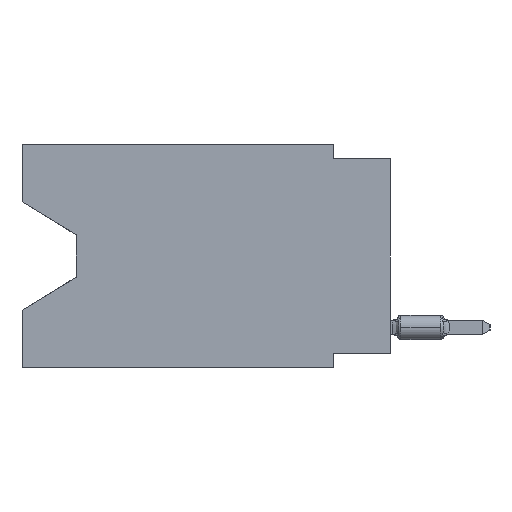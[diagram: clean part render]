
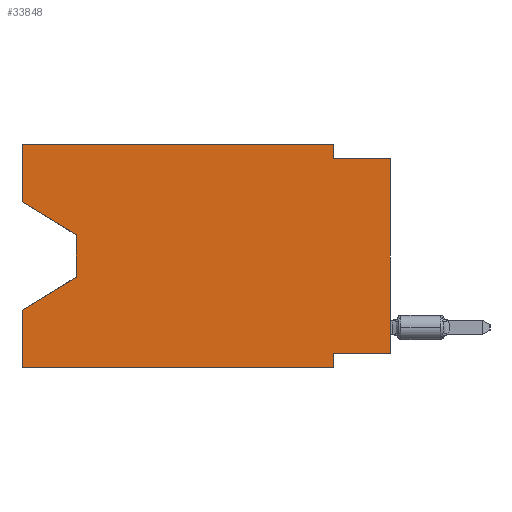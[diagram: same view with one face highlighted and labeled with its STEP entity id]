
A CAD part, left-side view. The second image highlights one B-rep face of the part: STEP entity #33848.
In plain terms, the highlighted planar face has unit normal (-1, 0, 0).
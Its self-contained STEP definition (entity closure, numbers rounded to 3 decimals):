
#257 = CARTESIAN_POINT ( 'NONE',  ( 0., 13.97, -5.893 ) ) ;
#1339 = VERTEX_POINT ( 'NONE', #38649 ) ;
#1725 = DIRECTION ( 'NONE',  ( 0., 0., -1. ) ) ;
#2882 = ORIENTED_EDGE ( 'NONE', *, *, #54597, .F. ) ;
#3100 = CARTESIAN_POINT ( 'NONE',  ( 0., 16.383, 0. ) ) ;
#3174 = VERTEX_POINT ( 'NONE', #54412 ) ;
#3651 = LINE ( 'NONE', #21540, #55730 ) ;
#3678 = DIRECTION ( 'NONE',  ( 0., 0., -1. ) ) ;
#3835 = CARTESIAN_POINT ( 'NONE',  ( 0., 0., -9.271 ) ) ;
#3837 = CARTESIAN_POINT ( 'NONE',  ( 0., 16.383, -2.546 ) ) ;
#4799 = VECTOR ( 'NONE', #37117, 1000. ) ;
#4942 = DIRECTION ( 'NONE',  ( 0., 0., -1. ) ) ;
#4967 = PLANE ( 'NONE',  #34024 ) ;
#5284 = CARTESIAN_POINT ( 'NONE',  ( 0., 16.383, 0. ) ) ;
#5517 = DIRECTION ( 'NONE',  ( 0., 0., -1. ) ) ;
#5522 = LINE ( 'NONE', #55066, #19893 ) ;
#5635 = ORIENTED_EDGE ( 'NONE', *, *, #6191, .T. ) ;
#6114 = DIRECTION ( 'NONE',  ( 1., 0., 0. ) ) ;
#6191 = EDGE_CURVE ( 'NONE', #15219, #54762, #33074, .T. ) ;
#6906 = VERTEX_POINT ( 'NONE', #33148 ) ;
#7361 = VECTOR ( 'NONE', #35498, 1000. ) ;
#8407 = LINE ( 'NONE', #13115, #34169 ) ;
#9062 = LINE ( 'NONE', #257, #13951 ) ;
#9277 = DIRECTION ( 'NONE',  ( 0., -1., 0. ) ) ;
#9693 = VECTOR ( 'NONE', #36617, 1000. ) ;
#9727 = EDGE_CURVE ( 'NONE', #12038, #9854, #42614, .T. ) ;
#9854 = VERTEX_POINT ( 'NONE', #57564 ) ;
#11542 = DIRECTION ( 'NONE',  ( 0., 0., 1. ) ) ;
#11933 = ORIENTED_EDGE ( 'NONE', *, *, #32653, .F. ) ;
#12038 = VERTEX_POINT ( 'NONE', #34923 ) ;
#12649 = LINE ( 'NONE', #3837, #7361 ) ;
#13115 = CARTESIAN_POINT ( 'NONE',  ( 0., 16.383, -9.906 ) ) ;
#13951 = VECTOR ( 'NONE', #54199, 1000. ) ;
#14295 = EDGE_CURVE ( 'NONE', #41225, #6906, #5522, .T. ) ;
#14967 = ORIENTED_EDGE ( 'NONE', *, *, #56402, .F. ) ;
#15132 = DIRECTION ( 'NONE',  ( 0., 0., 1. ) ) ;
#15219 = VERTEX_POINT ( 'NONE', #49995 ) ;
#15220 = DIRECTION ( 'NONE',  ( 0., -1., 0. ) ) ;
#15354 = CARTESIAN_POINT ( 'NONE',  ( 0., 16.383, 0. ) ) ;
#16816 = ORIENTED_EDGE ( 'NONE', *, *, #43141, .T. ) ;
#16878 = LINE ( 'NONE', #29773, #35104 ) ;
#18830 = EDGE_CURVE ( 'NONE', #38979, #1339, #3651, .T. ) ;
#19595 = FACE_OUTER_BOUND ( 'NONE', #54735, .T. ) ;
#19617 = LINE ( 'NONE', #5284, #39545 ) ;
#19893 = VECTOR ( 'NONE', #4942, 1000. ) ;
#20868 = LINE ( 'NONE', #3835, #57736 ) ;
#21540 = CARTESIAN_POINT ( 'NONE',  ( 0., 13.97, -4.013 ) ) ;
#21886 = VERTEX_POINT ( 'NONE', #40273 ) ;
#22890 = EDGE_CURVE ( 'NONE', #15219, #42087, #20868, .T. ) ;
#23347 = VECTOR ( 'NONE', #11542, 1000. ) ;
#24059 = VECTOR ( 'NONE', #15132, 1000. ) ;
#24498 = LINE ( 'NONE', #51465, #4799 ) ;
#25412 = EDGE_CURVE ( 'NONE', #3174, #54744, #42968, .T. ) ;
#26415 = ORIENTED_EDGE ( 'NONE', *, *, #44869, .T. ) ;
#27818 = CARTESIAN_POINT ( 'NONE',  ( 0., 16.383, 0. ) ) ;
#27942 = CARTESIAN_POINT ( 'NONE',  ( 0., 2.54, 0. ) ) ;
#29677 = ORIENTED_EDGE ( 'NONE', *, *, #9727, .F. ) ;
#29773 = CARTESIAN_POINT ( 'NONE',  ( 0., 2.54, -9.906 ) ) ;
#30940 = CARTESIAN_POINT ( 'NONE',  ( 0., 16.383, -7.36 ) ) ;
#32653 = EDGE_CURVE ( 'NONE', #6906, #54762, #24498, .T. ) ;
#32776 = CARTESIAN_POINT ( 'NONE',  ( 0., 0., 0. ) ) ;
#33074 = LINE ( 'NONE', #32776, #9693 ) ;
#33148 = CARTESIAN_POINT ( 'NONE',  ( 0., 2.54, -0.635 ) ) ;
#33848 = ADVANCED_FACE ( 'NONE', ( #19595 ), #4967, .F. ) ;
#34024 = AXIS2_PLACEMENT_3D ( 'NONE', #27818, #6114, #1725 ) ;
#34046 = DIRECTION ( 'NONE',  ( 0., 1., 0. ) ) ;
#34169 = VECTOR ( 'NONE', #9277, 1000. ) ;
#34923 = CARTESIAN_POINT ( 'NONE',  ( 0., 16.383, -2.546 ) ) ;
#35104 = VECTOR ( 'NONE', #3678, 1000. ) ;
#35489 = ORIENTED_EDGE ( 'NONE', *, *, #22890, .F. ) ;
#35498 = DIRECTION ( 'NONE',  ( 0., -0.855, -0.519 ) ) ;
#36617 = DIRECTION ( 'NONE',  ( 0., 0., 1. ) ) ;
#37117 = DIRECTION ( 'NONE',  ( 0., -1., 0. ) ) ;
#38112 = CARTESIAN_POINT ( 'NONE',  ( 0., 2.54, -9.271 ) ) ;
#38570 = ORIENTED_EDGE ( 'NONE', *, *, #18830, .T. ) ;
#38649 = CARTESIAN_POINT ( 'NONE',  ( 0., 13.97, -5.893 ) ) ;
#38979 = VERTEX_POINT ( 'NONE', #50953 ) ;
#39545 = VECTOR ( 'NONE', #15220, 1000. ) ;
#40273 = CARTESIAN_POINT ( 'NONE',  ( 0., 2.54, -9.906 ) ) ;
#40646 = EDGE_CURVE ( 'NONE', #3174, #21886, #8407, .T. ) ;
#41175 = ORIENTED_EDGE ( 'NONE', *, *, #25412, .F. ) ;
#41225 = VERTEX_POINT ( 'NONE', #27942 ) ;
#42087 = VERTEX_POINT ( 'NONE', #38112 ) ;
#42614 = LINE ( 'NONE', #15354, #23347 ) ;
#42968 = LINE ( 'NONE', #3100, #24059 ) ;
#43141 = EDGE_CURVE ( 'NONE', #1339, #54744, #9062, .T. ) ;
#44869 = EDGE_CURVE ( 'NONE', #12038, #38979, #12649, .T. ) ;
#49995 = CARTESIAN_POINT ( 'NONE',  ( 0., 0., -9.271 ) ) ;
#50772 = ORIENTED_EDGE ( 'NONE', *, *, #40646, .T. ) ;
#50953 = CARTESIAN_POINT ( 'NONE',  ( 0., 13.97, -4.013 ) ) ;
#51465 = CARTESIAN_POINT ( 'NONE',  ( 0., 0., -0.635 ) ) ;
#51569 = CARTESIAN_POINT ( 'NONE',  ( 0., 0., -0.635 ) ) ;
#54199 = DIRECTION ( 'NONE',  ( 0., 0.855, -0.519 ) ) ;
#54412 = CARTESIAN_POINT ( 'NONE',  ( 0., 16.383, -9.906 ) ) ;
#54597 = EDGE_CURVE ( 'NONE', #9854, #41225, #19617, .T. ) ;
#54735 = EDGE_LOOP ( 'NONE', ( #26415, #38570, #16816, #41175, #50772, #14967, #35489, #5635, #11933, #56081, #2882, #29677 ) ) ;
#54744 = VERTEX_POINT ( 'NONE', #30940 ) ;
#54762 = VERTEX_POINT ( 'NONE', #51569 ) ;
#55066 = CARTESIAN_POINT ( 'NONE',  ( 0., 2.54, 0. ) ) ;
#55730 = VECTOR ( 'NONE', #5517, 1000. ) ;
#56081 = ORIENTED_EDGE ( 'NONE', *, *, #14295, .F. ) ;
#56402 = EDGE_CURVE ( 'NONE', #42087, #21886, #16878, .T. ) ;
#57564 = CARTESIAN_POINT ( 'NONE',  ( 0., 16.383, 0. ) ) ;
#57736 = VECTOR ( 'NONE', #34046, 1000. ) ;
